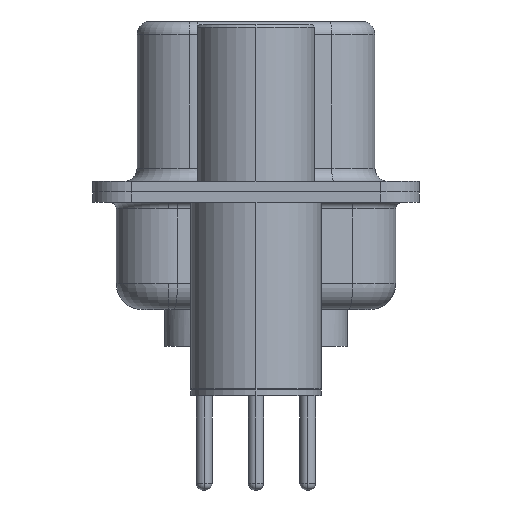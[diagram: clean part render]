
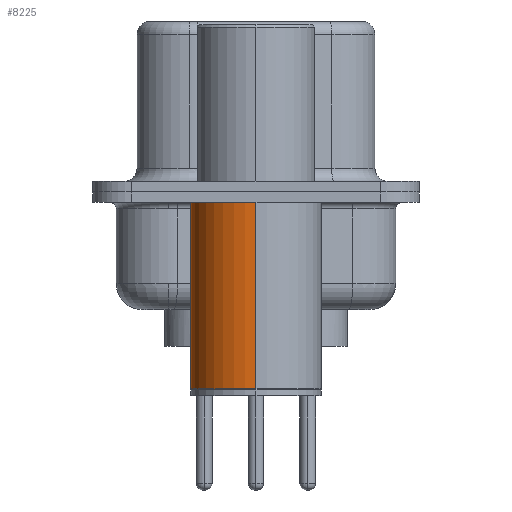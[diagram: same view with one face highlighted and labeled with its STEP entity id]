
A CAD part, left-side view. The second image highlights one B-rep face of the part: STEP entity #8225.
In plain terms, the highlighted cylindrical face has radius 2.5 mm (diameter 5 mm), a partial arc.
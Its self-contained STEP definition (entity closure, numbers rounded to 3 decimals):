
#1095 = CARTESIAN_POINT ( 'NONE',  ( -2.5, 0., -7.525 ) ) ;
#2048 = LINE ( 'NONE', #20022, #14893 ) ;
#2631 = CARTESIAN_POINT ( 'NONE',  ( 0., 0., -0.4 ) ) ;
#4030 = EDGE_CURVE ( 'NONE', #18217, #20069, #22369, .T. ) ;
#4302 = AXIS2_PLACEMENT_3D ( 'NONE', #2631, #14852, #4401 ) ;
#4318 = EDGE_CURVE ( 'NONE', #5990, #18217, #16433, .T. ) ;
#4401 = DIRECTION ( 'NONE',  ( 1., 0., 0. ) ) ;
#4675 = CARTESIAN_POINT ( 'NONE',  ( -2.5, 0., -0.4 ) ) ;
#4781 = EDGE_LOOP ( 'NONE', ( #19478, #8775, #22386, #21952 ) ) ;
#5731 = CIRCLE ( 'NONE', #4302, 2.5 ) ;
#5990 = VERTEX_POINT ( 'NONE', #16246 ) ;
#6932 = CARTESIAN_POINT ( 'NONE',  ( -2.5, 0., 0.581 ) ) ;
#7171 = DIRECTION ( 'NONE',  ( 0., 0., 1. ) ) ;
#8225 = ADVANCED_FACE ( 'NONE', ( #19799 ), #15215, .T. ) ;
#8775 = ORIENTED_EDGE ( 'NONE', *, *, #4030, .T. ) ;
#9716 = EDGE_CURVE ( 'NONE', #5990, #13364, #2048, .T. ) ;
#11413 = DIRECTION ( 'NONE',  ( 0., 0., 1. ) ) ;
#13307 = CARTESIAN_POINT ( 'NONE',  ( 0., 0., 0.581 ) ) ;
#13364 = VERTEX_POINT ( 'NONE', #16578 ) ;
#14676 = EDGE_CURVE ( 'NONE', #13364, #20069, #5731, .T. ) ;
#14852 = DIRECTION ( 'NONE',  ( 0., 0., 1. ) ) ;
#14893 = VECTOR ( 'NONE', #11413, 1000. ) ;
#15215 = CYLINDRICAL_SURFACE ( 'NONE', #18352, 2.5 ) ;
#16246 = CARTESIAN_POINT ( 'NONE',  ( 2.5, 0., -7.525 ) ) ;
#16433 = CIRCLE ( 'NONE', #18298, 2.5 ) ;
#16578 = CARTESIAN_POINT ( 'NONE',  ( 2.5, 0., -0.4 ) ) ;
#16712 = VECTOR ( 'NONE', #7171, 1000. ) ;
#16767 = DIRECTION ( 'NONE',  ( 0., 0., 1. ) ) ;
#18217 = VERTEX_POINT ( 'NONE', #1095 ) ;
#18298 = AXIS2_PLACEMENT_3D ( 'NONE', #21927, #21122, #21120 ) ;
#18352 = AXIS2_PLACEMENT_3D ( 'NONE', #13307, #16767, #18487 ) ;
#18487 = DIRECTION ( 'NONE',  ( 1., 0., 0. ) ) ;
#19478 = ORIENTED_EDGE ( 'NONE', *, *, #4318, .T. ) ;
#19799 = FACE_OUTER_BOUND ( 'NONE', #4781, .T. ) ;
#20022 = CARTESIAN_POINT ( 'NONE',  ( 2.5, 0., 0.581 ) ) ;
#20069 = VERTEX_POINT ( 'NONE', #4675 ) ;
#21120 = DIRECTION ( 'NONE',  ( 1., 0., 0. ) ) ;
#21122 = DIRECTION ( 'NONE',  ( 0., 0., 1. ) ) ;
#21927 = CARTESIAN_POINT ( 'NONE',  ( 0., 0., -7.525 ) ) ;
#21952 = ORIENTED_EDGE ( 'NONE', *, *, #9716, .F. ) ;
#22369 = LINE ( 'NONE', #6932, #16712 ) ;
#22386 = ORIENTED_EDGE ( 'NONE', *, *, #14676, .F. ) ;
